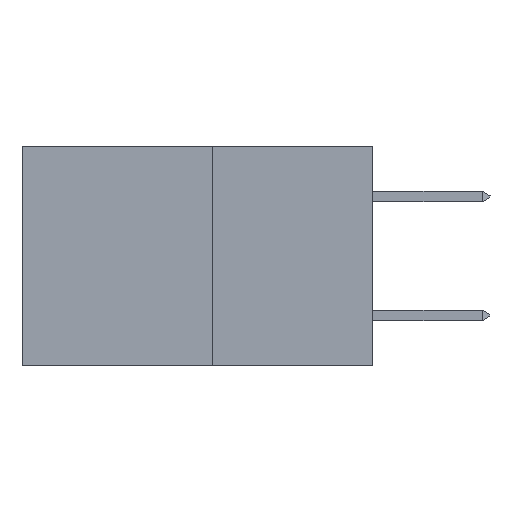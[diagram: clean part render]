
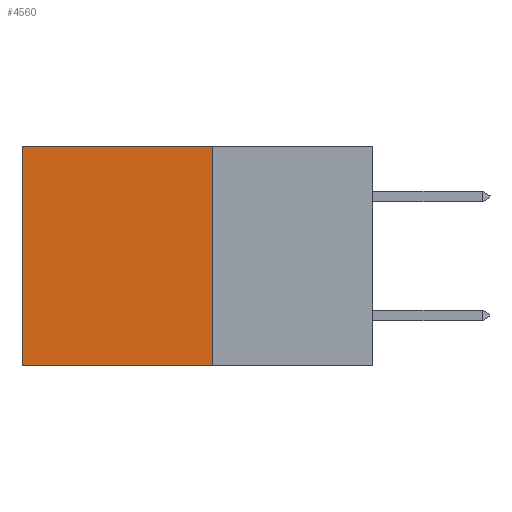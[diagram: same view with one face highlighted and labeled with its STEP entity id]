
A CAD part, left-side view. The second image highlights one B-rep face of the part: STEP entity #4560.
In plain terms, the highlighted planar face has unit normal (-1, 0, 0).
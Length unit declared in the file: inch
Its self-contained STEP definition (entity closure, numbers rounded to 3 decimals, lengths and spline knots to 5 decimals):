
#21 = VECTOR ( 'NONE', #1865, 39.37008 ) ;
#1500 = DIRECTION ( 'NONE',  ( 0., 0., -1. ) ) ;
#1865 = DIRECTION ( 'NONE',  ( 0., 1., 0. ) ) ;
#2496 = CARTESIAN_POINT ( 'NONE',  ( 0.277, 0.27, -0.37 ) ) ;
#2550 = VECTOR ( 'NONE', #1500, 39.37008 ) ;
#3265 = LINE ( 'NONE', #25234, #8243 ) ;
#3452 = CARTESIAN_POINT ( 'NONE',  ( 0.277, 0.59, -0.37 ) ) ;
#3686 = ORIENTED_EDGE ( 'NONE', *, *, #6450, .F. ) ;
#4560 = ADVANCED_FACE ( 'NONE', ( #17464 ), #22613, .F. ) ;
#6339 = VERTEX_POINT ( 'NONE', #9478 ) ;
#6450 = EDGE_CURVE ( 'NONE', #6339, #15842, #11232, .T. ) ;
#8243 = VECTOR ( 'NONE', #8520, 39.37008 ) ;
#8520 = DIRECTION ( 'NONE',  ( 0., 1., 0. ) ) ;
#8713 = VERTEX_POINT ( 'NONE', #3452 ) ;
#9478 = CARTESIAN_POINT ( 'NONE',  ( 0.277, 0.27, 0. ) ) ;
#10897 = LINE ( 'NONE', #14407, #21 ) ;
#11232 = LINE ( 'NONE', #18254, #22328 ) ;
#11936 = DIRECTION ( 'NONE',  ( 0., 0., -1. ) ) ;
#13584 = CARTESIAN_POINT ( 'NONE',  ( 0.277, 0.59, 0. ) ) ;
#13940 = EDGE_CURVE ( 'NONE', #15842, #8713, #3265, .T. ) ;
#14362 = EDGE_LOOP ( 'NONE', ( #25202, #23998, #3686, #16469 ) ) ;
#14407 = CARTESIAN_POINT ( 'NONE',  ( 0.277, 0.27, 0. ) ) ;
#14545 = AXIS2_PLACEMENT_3D ( 'NONE', #22648, #22285, #21951 ) ;
#14814 = EDGE_CURVE ( 'NONE', #23361, #8713, #19268, .T. ) ;
#15842 = VERTEX_POINT ( 'NONE', #2496 ) ;
#16469 = ORIENTED_EDGE ( 'NONE', *, *, #24370, .T. ) ;
#17464 = FACE_OUTER_BOUND ( 'NONE', #14362, .T. ) ;
#18254 = CARTESIAN_POINT ( 'NONE',  ( 0.277, 0.27, -0.37 ) ) ;
#19268 = LINE ( 'NONE', #26641, #2550 ) ;
#21951 = DIRECTION ( 'NONE',  ( 0., 0., -1. ) ) ;
#22285 = DIRECTION ( 'NONE',  ( 1., 0., 0. ) ) ;
#22328 = VECTOR ( 'NONE', #11936, 39.37008 ) ;
#22613 = PLANE ( 'NONE',  #14545 ) ;
#22648 = CARTESIAN_POINT ( 'NONE',  ( 0.277, 0.27, -0.37 ) ) ;
#23361 = VERTEX_POINT ( 'NONE', #13584 ) ;
#23998 = ORIENTED_EDGE ( 'NONE', *, *, #13940, .F. ) ;
#24370 = EDGE_CURVE ( 'NONE', #6339, #23361, #10897, .T. ) ;
#25202 = ORIENTED_EDGE ( 'NONE', *, *, #14814, .T. ) ;
#25234 = CARTESIAN_POINT ( 'NONE',  ( 0.277, 0.27, -0.37 ) ) ;
#26641 = CARTESIAN_POINT ( 'NONE',  ( 0.277, 0.59, -0.37 ) ) ;
